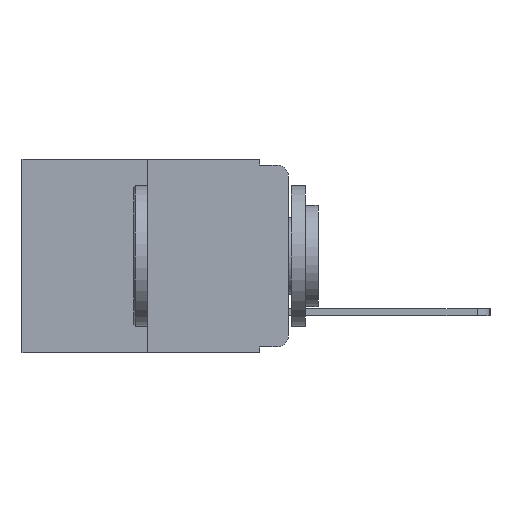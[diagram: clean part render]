
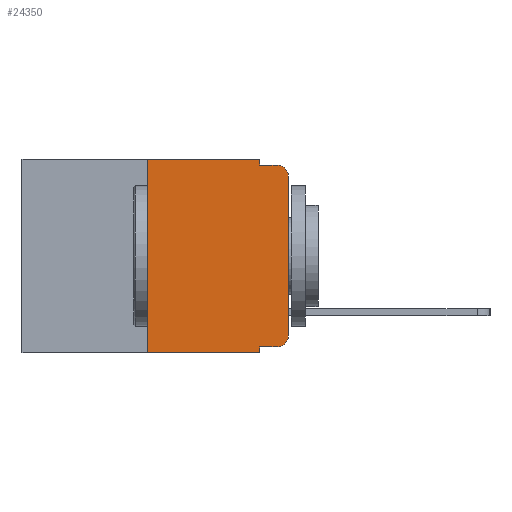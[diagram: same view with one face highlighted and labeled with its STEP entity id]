
A CAD part, left-side view. The second image highlights one B-rep face of the part: STEP entity #24350.
In plain terms, the highlighted planar face has unit normal (-1, 0, 0).
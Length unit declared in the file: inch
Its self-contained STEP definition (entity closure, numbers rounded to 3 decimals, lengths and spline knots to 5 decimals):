
#20 = VECTOR ( 'NONE', #12700, 39.37008 ) ;
#159 = VECTOR ( 'NONE', #14753, 39.37008 ) ;
#338 = VERTEX_POINT ( 'NONE', #10116 ) ;
#682 = DIRECTION ( 'NONE',  ( -1., 0., 0. ) ) ;
#908 = DIRECTION ( 'NONE',  ( 0., 0., -1. ) ) ;
#1577 = VERTEX_POINT ( 'NONE', #10054 ) ;
#2259 = DIRECTION ( 'NONE',  ( 0., -1., 0. ) ) ;
#2318 = CIRCLE ( 'NONE', #3192, 0.02 ) ;
#2497 = VERTEX_POINT ( 'NONE', #24719 ) ;
#2536 = FACE_OUTER_BOUND ( 'NONE', #19899, .T. ) ;
#2545 = AXIS2_PLACEMENT_3D ( 'NONE', #12382, #682, #14349 ) ;
#2623 = EDGE_CURVE ( 'NONE', #11763, #338, #10417, .T. ) ;
#3192 = AXIS2_PLACEMENT_3D ( 'NONE', #21249, #9682, #23186 ) ;
#3919 = EDGE_CURVE ( 'NONE', #5787, #24899, #21219, .T. ) ;
#4321 = CARTESIAN_POINT ( 'NONE',  ( 0., 0.051, 0. ) ) ;
#4485 = ORIENTED_EDGE ( 'NONE', *, *, #4603, .F. ) ;
#4603 = EDGE_CURVE ( 'NONE', #1577, #2497, #14556, .T. ) ;
#4996 = DIRECTION ( 'NONE',  ( 0., 0., -1. ) ) ;
#5050 = VERTEX_POINT ( 'NONE', #11164 ) ;
#5466 = EDGE_CURVE ( 'NONE', #24899, #18712, #6011, .T. ) ;
#5755 = DIRECTION ( 'NONE',  ( 0., 0., 1. ) ) ;
#5787 = VERTEX_POINT ( 'NONE', #18938 ) ;
#6011 = LINE ( 'NONE', #12703, #159 ) ;
#6697 = ORIENTED_EDGE ( 'NONE', *, *, #12528, .T. ) ;
#6902 = PLANE ( 'NONE',  #15376 ) ;
#6905 = DIRECTION ( 'NONE',  ( 0., -1., 0. ) ) ;
#7000 = CARTESIAN_POINT ( 'NONE',  ( 0., 0., -0.03 ) ) ;
#7191 = DIRECTION ( 'NONE',  ( 0., 0., -1. ) ) ;
#8495 = VECTOR ( 'NONE', #2259, 39.37008 ) ;
#8521 = LINE ( 'NONE', #19280, #9142 ) ;
#8616 = VERTEX_POINT ( 'NONE', #7000 ) ;
#8879 = ORIENTED_EDGE ( 'NONE', *, *, #16783, .T. ) ;
#9102 = LINE ( 'NONE', #22336, #13649 ) ;
#9142 = VECTOR ( 'NONE', #5755, 39.37008 ) ;
#9410 = VECTOR ( 'NONE', #23273, 39.37008 ) ;
#9682 = DIRECTION ( 'NONE',  ( -1., 0., 0. ) ) ;
#9996 = ORIENTED_EDGE ( 'NONE', *, *, #3919, .F. ) ;
#10054 = CARTESIAN_POINT ( 'NONE',  ( 0., 0.25, -0.343 ) ) ;
#10116 = CARTESIAN_POINT ( 'NONE',  ( 0., 0.02, -0.333 ) ) ;
#10417 = LINE ( 'NONE', #13164, #20 ) ;
#10744 = ORIENTED_EDGE ( 'NONE', *, *, #5466, .F. ) ;
#10790 = CARTESIAN_POINT ( 'NONE',  ( 0., 0.473, 0. ) ) ;
#11164 = CARTESIAN_POINT ( 'NONE',  ( 0., 0., -0.313 ) ) ;
#11763 = VERTEX_POINT ( 'NONE', #17492 ) ;
#12382 = CARTESIAN_POINT ( 'NONE',  ( 0., 0.02, -0.03 ) ) ;
#12528 = EDGE_CURVE ( 'NONE', #1577, #15974, #9102, .T. ) ;
#12600 = CARTESIAN_POINT ( 'NONE',  ( 0., 0.051, 0. ) ) ;
#12700 = DIRECTION ( 'NONE',  ( 0., -1., 0. ) ) ;
#12703 = CARTESIAN_POINT ( 'NONE',  ( 0., 0.051, -0.01 ) ) ;
#13164 = CARTESIAN_POINT ( 'NONE',  ( 0., 0.051, -0.333 ) ) ;
#13649 = VECTOR ( 'NONE', #6905, 39.37008 ) ;
#14349 = DIRECTION ( 'NONE',  ( 0., 0., -1. ) ) ;
#14556 = LINE ( 'NONE', #23803, #9410 ) ;
#14676 = CARTESIAN_POINT ( 'NONE',  ( 0., 0.051, -0.01 ) ) ;
#14753 = DIRECTION ( 'NONE',  ( 0., -1., 0. ) ) ;
#14822 = VECTOR ( 'NONE', #908, 39.37008 ) ;
#15376 = AXIS2_PLACEMENT_3D ( 'NONE', #10790, #16603, #4996 ) ;
#15644 = EDGE_CURVE ( 'NONE', #5050, #8616, #8521, .T. ) ;
#15974 = VERTEX_POINT ( 'NONE', #16828 ) ;
#16085 = VECTOR ( 'NONE', #7191, 39.37008 ) ;
#16144 = ORIENTED_EDGE ( 'NONE', *, *, #15644, .T. ) ;
#16603 = DIRECTION ( 'NONE',  ( 1., 0., 0. ) ) ;
#16783 = EDGE_CURVE ( 'NONE', #338, #5050, #2318, .T. ) ;
#16828 = CARTESIAN_POINT ( 'NONE',  ( 0., 0.051, -0.343 ) ) ;
#16883 = EDGE_CURVE ( 'NONE', #11763, #15974, #24981, .T. ) ;
#17492 = CARTESIAN_POINT ( 'NONE',  ( 0., 0.051, -0.333 ) ) ;
#17936 = EDGE_CURVE ( 'NONE', #8616, #18712, #24649, .T. ) ;
#18156 = ORIENTED_EDGE ( 'NONE', *, *, #16883, .F. ) ;
#18712 = VERTEX_POINT ( 'NONE', #24373 ) ;
#18732 = LINE ( 'NONE', #23439, #8495 ) ;
#18938 = CARTESIAN_POINT ( 'NONE',  ( 0., 0.051, 0. ) ) ;
#19280 = CARTESIAN_POINT ( 'NONE',  ( 0., 0., 0. ) ) ;
#19899 = EDGE_LOOP ( 'NONE', ( #16144, #20698, #10744, #9996, #23852, #4485, #6697, #18156, #25071, #8879 ) ) ;
#20698 = ORIENTED_EDGE ( 'NONE', *, *, #17936, .T. ) ;
#21219 = LINE ( 'NONE', #4321, #16085 ) ;
#21249 = CARTESIAN_POINT ( 'NONE',  ( 0., 0.02, -0.313 ) ) ;
#22152 = EDGE_CURVE ( 'NONE', #2497, #5787, #18732, .T. ) ;
#22336 = CARTESIAN_POINT ( 'NONE',  ( 0., 0.473, -0.343 ) ) ;
#23186 = DIRECTION ( 'NONE',  ( 0., 0., -1. ) ) ;
#23273 = DIRECTION ( 'NONE',  ( 0., 0., 1. ) ) ;
#23439 = CARTESIAN_POINT ( 'NONE',  ( 0., 0.473, 0. ) ) ;
#23803 = CARTESIAN_POINT ( 'NONE',  ( 0., 0.25, 0. ) ) ;
#23852 = ORIENTED_EDGE ( 'NONE', *, *, #22152, .F. ) ;
#24350 = ADVANCED_FACE ( 'NONE', ( #2536 ), #6902, .F. ) ;
#24373 = CARTESIAN_POINT ( 'NONE',  ( 0., 0.02, -0.01 ) ) ;
#24649 = CIRCLE ( 'NONE', #2545, 0.02 ) ;
#24719 = CARTESIAN_POINT ( 'NONE',  ( 0., 0.25, 0. ) ) ;
#24899 = VERTEX_POINT ( 'NONE', #14676 ) ;
#24981 = LINE ( 'NONE', #12600, #14822 ) ;
#25071 = ORIENTED_EDGE ( 'NONE', *, *, #2623, .T. ) ;
